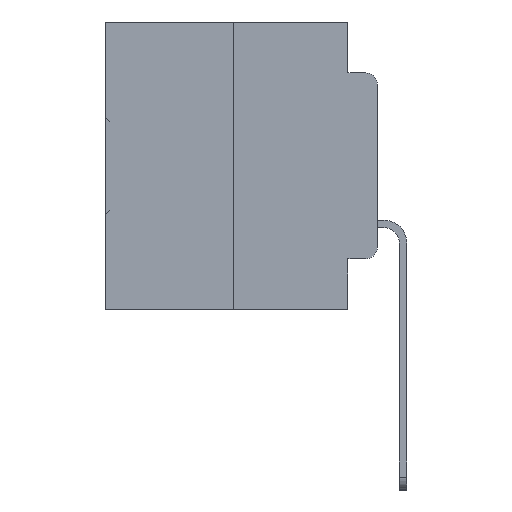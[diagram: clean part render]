
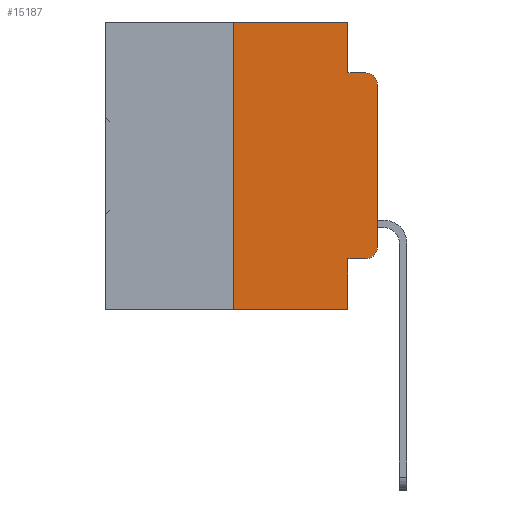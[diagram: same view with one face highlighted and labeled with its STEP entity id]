
A CAD part, left-side view. The second image highlights one B-rep face of the part: STEP entity #15187.
In plain terms, the highlighted planar face has unit normal (-1, 0, 0).
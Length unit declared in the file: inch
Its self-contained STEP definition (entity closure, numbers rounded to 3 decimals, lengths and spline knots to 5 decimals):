
#479 = EDGE_CURVE ( 'NONE', #7359, #19543, #9970, .T. ) ;
#593 = CARTESIAN_POINT ( 'NONE',  ( 0., 0.051, 0. ) ) ;
#934 = VECTOR ( 'NONE', #31480, 39.37008 ) ;
#935 = AXIS2_PLACEMENT_3D ( 'NONE', #7618, #27107, #10425 ) ;
#1476 = DIRECTION ( 'NONE',  ( 0., -1., 0. ) ) ;
#1546 = CARTESIAN_POINT ( 'NONE',  ( 0., 0., 0. ) ) ;
#1980 = LINE ( 'NONE', #13905, #31055 ) ;
#3097 = LINE ( 'NONE', #3544, #17306 ) ;
#3544 = CARTESIAN_POINT ( 'NONE',  ( 0., 0.473, -0.5 ) ) ;
#3819 = LINE ( 'NONE', #7484, #10567 ) ;
#4231 = LINE ( 'NONE', #35230, #32257 ) ;
#4430 = DIRECTION ( 'NONE',  ( -1., 0., 0. ) ) ;
#4850 = ORIENTED_EDGE ( 'NONE', *, *, #21845, .T. ) ;
#5224 = CARTESIAN_POINT ( 'NONE',  ( 0., 0., -0.3915 ) ) ;
#5484 = DIRECTION ( 'NONE',  ( 0., -1., 0. ) ) ;
#6651 = DIRECTION ( 'NONE',  ( 0., -1., 0. ) ) ;
#6785 = EDGE_CURVE ( 'NONE', #7359, #14654, #3097, .T. ) ;
#7071 = FACE_OUTER_BOUND ( 'NONE', #28937, .T. ) ;
#7212 = ORIENTED_EDGE ( 'NONE', *, *, #23280, .F. ) ;
#7359 = VERTEX_POINT ( 'NONE', #22703 ) ;
#7484 = CARTESIAN_POINT ( 'NONE',  ( 0., 0.051, -0.0885 ) ) ;
#7498 = DIRECTION ( 'NONE',  ( 0., 0., 1. ) ) ;
#7618 = CARTESIAN_POINT ( 'NONE',  ( 0., 0.02, -0.3915 ) ) ;
#8283 = DIRECTION ( 'NONE',  ( 0., 0., -1. ) ) ;
#8716 = DIRECTION ( 'NONE',  ( 0., 0., -1. ) ) ;
#9596 = VERTEX_POINT ( 'NONE', #19010 ) ;
#9963 = ORIENTED_EDGE ( 'NONE', *, *, #31131, .T. ) ;
#9970 = LINE ( 'NONE', #10706, #35988 ) ;
#10269 = ORIENTED_EDGE ( 'NONE', *, *, #6785, .T. ) ;
#10297 = DIRECTION ( 'NONE',  ( 0., -1., 0. ) ) ;
#10425 = DIRECTION ( 'NONE',  ( 0., 0., -1. ) ) ;
#10567 = VECTOR ( 'NONE', #10297, 39.37008 ) ;
#10636 = CARTESIAN_POINT ( 'NONE',  ( 0., 0.051, -0.5 ) ) ;
#10706 = CARTESIAN_POINT ( 'NONE',  ( 0., 0.25, 0. ) ) ;
#10960 = VECTOR ( 'NONE', #8716, 39.37008 ) ;
#11476 = CARTESIAN_POINT ( 'NONE',  ( 0., 0.25, 0. ) ) ;
#11505 = EDGE_CURVE ( 'NONE', #19625, #19177, #25202, .T. ) ;
#11615 = ORIENTED_EDGE ( 'NONE', *, *, #16462, .F. ) ;
#12898 = ORIENTED_EDGE ( 'NONE', *, *, #22647, .F. ) ;
#13905 = CARTESIAN_POINT ( 'NONE',  ( 0., 0.051, -0.4115 ) ) ;
#14654 = VERTEX_POINT ( 'NONE', #10636 ) ;
#15187 = ADVANCED_FACE ( 'NONE', ( #7071 ), #35935, .F. ) ;
#15370 = DIRECTION ( 'NONE',  ( 0., 0., 1. ) ) ;
#15502 = ORIENTED_EDGE ( 'NONE', *, *, #479, .F. ) ;
#15532 = AXIS2_PLACEMENT_3D ( 'NONE', #27655, #24976, #8283 ) ;
#15742 = ORIENTED_EDGE ( 'NONE', *, *, #11505, .T. ) ;
#16462 = EDGE_CURVE ( 'NONE', #27233, #14654, #31798, .T. ) ;
#16940 = VECTOR ( 'NONE', #7498, 39.37008 ) ;
#17306 = VECTOR ( 'NONE', #6651, 39.37008 ) ;
#17608 = EDGE_CURVE ( 'NONE', #27233, #24256, #1980, .T. ) ;
#18855 = CARTESIAN_POINT ( 'NONE',  ( 0., 0.02, -0.0885 ) ) ;
#19010 = CARTESIAN_POINT ( 'NONE',  ( 0., 0.051, -0.0885 ) ) ;
#19177 = VERTEX_POINT ( 'NONE', #34754 ) ;
#19543 = VERTEX_POINT ( 'NONE', #11476 ) ;
#19625 = VERTEX_POINT ( 'NONE', #5224 ) ;
#21250 = CARTESIAN_POINT ( 'NONE',  ( 0., 0.02, -0.1085 ) ) ;
#21294 = VERTEX_POINT ( 'NONE', #18855 ) ;
#21845 = EDGE_CURVE ( 'NONE', #19177, #21294, #30539, .T. ) ;
#22428 = CIRCLE ( 'NONE', #935, 0.02 ) ;
#22647 = EDGE_CURVE ( 'NONE', #9596, #21294, #3819, .T. ) ;
#22703 = CARTESIAN_POINT ( 'NONE',  ( 0., 0.25, -0.5 ) ) ;
#23072 = VERTEX_POINT ( 'NONE', #593 ) ;
#23280 = EDGE_CURVE ( 'NONE', #19543, #23072, #4231, .T. ) ;
#23616 = CARTESIAN_POINT ( 'NONE',  ( 0., 0.051, -0.4115 ) ) ;
#24076 = DIRECTION ( 'NONE',  ( 0., 0., -1. ) ) ;
#24256 = VERTEX_POINT ( 'NONE', #25175 ) ;
#24976 = DIRECTION ( 'NONE',  ( 1., 0., 0. ) ) ;
#25175 = CARTESIAN_POINT ( 'NONE',  ( 0., 0.02, -0.4115 ) ) ;
#25202 = LINE ( 'NONE', #1546, #16940 ) ;
#25773 = LINE ( 'NONE', #33618, #10960 ) ;
#26869 = ORIENTED_EDGE ( 'NONE', *, *, #17608, .T. ) ;
#27107 = DIRECTION ( 'NONE',  ( -1., 0., 0. ) ) ;
#27233 = VERTEX_POINT ( 'NONE', #23616 ) ;
#27655 = CARTESIAN_POINT ( 'NONE',  ( 0., 0.473, 0. ) ) ;
#28709 = CARTESIAN_POINT ( 'NONE',  ( 0., 0.051, 0. ) ) ;
#28937 = EDGE_LOOP ( 'NONE', ( #15742, #4850, #12898, #34566, #7212, #15502, #10269, #11615, #26869, #9963 ) ) ;
#30539 = CIRCLE ( 'NONE', #31951, 0.02 ) ;
#31055 = VECTOR ( 'NONE', #5484, 39.37008 ) ;
#31131 = EDGE_CURVE ( 'NONE', #24256, #19625, #22428, .T. ) ;
#31480 = DIRECTION ( 'NONE',  ( 0., 0., -1. ) ) ;
#31798 = LINE ( 'NONE', #28709, #934 ) ;
#31951 = AXIS2_PLACEMENT_3D ( 'NONE', #21250, #4430, #24076 ) ;
#32257 = VECTOR ( 'NONE', #1476, 39.37008 ) ;
#33122 = EDGE_CURVE ( 'NONE', #23072, #9596, #25773, .T. ) ;
#33618 = CARTESIAN_POINT ( 'NONE',  ( 0., 0.051, 0. ) ) ;
#34566 = ORIENTED_EDGE ( 'NONE', *, *, #33122, .F. ) ;
#34754 = CARTESIAN_POINT ( 'NONE',  ( 0., 0., -0.1085 ) ) ;
#35230 = CARTESIAN_POINT ( 'NONE',  ( 0., 0.473, 0. ) ) ;
#35935 = PLANE ( 'NONE',  #15532 ) ;
#35988 = VECTOR ( 'NONE', #15370, 39.37008 ) ;
